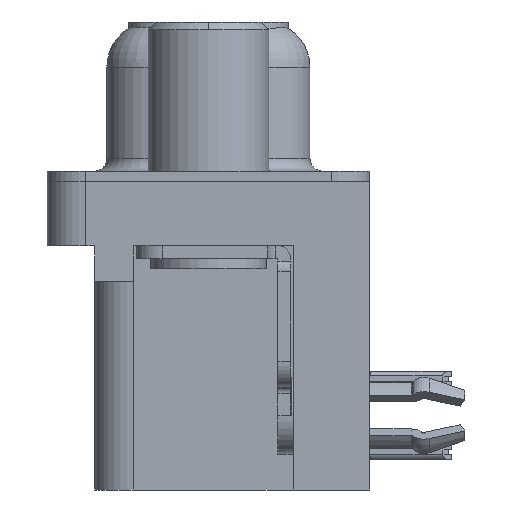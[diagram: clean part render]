
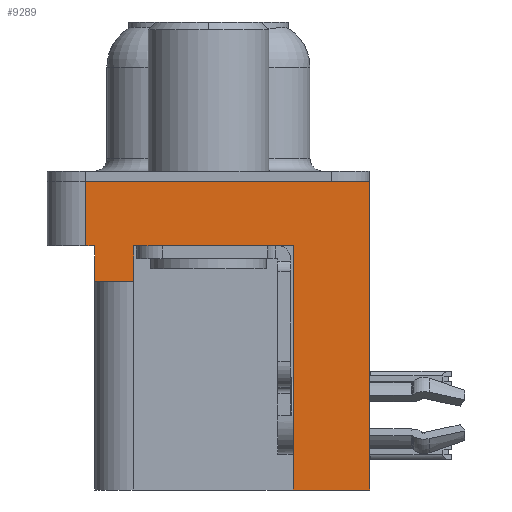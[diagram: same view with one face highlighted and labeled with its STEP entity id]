
A CAD part, left-side view. The second image highlights one B-rep face of the part: STEP entity #9289.
In plain terms, the highlighted planar face has unit normal (-1, 0, 0).
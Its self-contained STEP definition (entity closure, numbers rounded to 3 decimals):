
#329 = CARTESIAN_POINT ( 'NONE',  ( -2.935, -3.295, -12. ) ) ;
#2155 = CARTESIAN_POINT ( 'NONE',  ( -2.935, -6.275, -2.5 ) ) ;
#2458 = VECTOR ( 'NONE', #23388, 1000. ) ;
#2579 = LINE ( 'NONE', #3087, #22049 ) ;
#2972 = VERTEX_POINT ( 'NONE', #27534 ) ;
#3087 = CARTESIAN_POINT ( 'NONE',  ( -2.935, 4.425, -3.9 ) ) ;
#3257 = DIRECTION ( 'NONE',  ( 0., -1., 0. ) ) ;
#3308 = LINE ( 'NONE', #10274, #9508 ) ;
#3377 = VERTEX_POINT ( 'NONE', #11298 ) ;
#3486 = VECTOR ( 'NONE', #20382, 1000. ) ;
#4013 = VERTEX_POINT ( 'NONE', #5230 ) ;
#4302 = FACE_OUTER_BOUND ( 'NONE', #19098, .T. ) ;
#4414 = CARTESIAN_POINT ( 'NONE',  ( -2.935, -6.275, -2.5 ) ) ;
#4572 = DIRECTION ( 'NONE',  ( 0., -1., 0. ) ) ;
#4605 = EDGE_CURVE ( 'NONE', #3377, #26899, #18835, .T. ) ;
#5190 = VERTEX_POINT ( 'NONE', #20100 ) ;
#5230 = CARTESIAN_POINT ( 'NONE',  ( -2.935, 2.895, -2.5 ) ) ;
#5231 = VERTEX_POINT ( 'NONE', #13754 ) ;
#6147 = ORIENTED_EDGE ( 'NONE', *, *, #16762, .F. ) ;
#6730 = VERTEX_POINT ( 'NONE', #24211 ) ;
#7639 = VERTEX_POINT ( 'NONE', #17720 ) ;
#7646 = DIRECTION ( 'NONE',  ( 0., 0., 1. ) ) ;
#8039 = LINE ( 'NONE', #27539, #25761 ) ;
#8700 = EDGE_CURVE ( 'NONE', #5190, #7639, #2579, .T. ) ;
#8951 = CARTESIAN_POINT ( 'NONE',  ( -2.935, -6.275, 0. ) ) ;
#9289 = ADVANCED_FACE ( 'NONE', ( #4302 ), #15103, .T. ) ;
#9508 = VECTOR ( 'NONE', #16993, 1000. ) ;
#9856 = LINE ( 'NONE', #4414, #21050 ) ;
#10104 = CARTESIAN_POINT ( 'NONE',  ( -2.935, -3.295, -2.5 ) ) ;
#10274 = CARTESIAN_POINT ( 'NONE',  ( -2.935, 4.775, -2.5 ) ) ;
#10456 = DIRECTION ( 'NONE',  ( 0., 1., 0. ) ) ;
#10618 = ORIENTED_EDGE ( 'NONE', *, *, #15160, .T. ) ;
#10689 = DIRECTION ( 'NONE',  ( -1., 0., 0. ) ) ;
#11298 = CARTESIAN_POINT ( 'NONE',  ( -2.935, 4.775, 0. ) ) ;
#11533 = ORIENTED_EDGE ( 'NONE', *, *, #8700, .F. ) ;
#11577 = CARTESIAN_POINT ( 'NONE',  ( -2.935, -3.295, -12. ) ) ;
#12272 = DIRECTION ( 'NONE',  ( 0., 0., 1. ) ) ;
#12697 = EDGE_CURVE ( 'NONE', #5231, #27297, #23297, .T. ) ;
#12913 = VECTOR ( 'NONE', #4572, 1000. ) ;
#13441 = CARTESIAN_POINT ( 'NONE',  ( -2.935, 2.895, -3.9 ) ) ;
#13754 = CARTESIAN_POINT ( 'NONE',  ( -2.935, -6.275, -12. ) ) ;
#14406 = ORIENTED_EDGE ( 'NONE', *, *, #17805, .F. ) ;
#14420 = ORIENTED_EDGE ( 'NONE', *, *, #26349, .F. ) ;
#14487 = LINE ( 'NONE', #13441, #20780 ) ;
#14980 = LINE ( 'NONE', #2155, #2458 ) ;
#15103 = PLANE ( 'NONE',  #15478 ) ;
#15160 = EDGE_CURVE ( 'NONE', #2972, #4013, #14487, .T. ) ;
#15478 = AXIS2_PLACEMENT_3D ( 'NONE', #19555, #10689, #28091 ) ;
#15591 = EDGE_CURVE ( 'NONE', #5231, #26899, #14980, .T. ) ;
#15917 = ORIENTED_EDGE ( 'NONE', *, *, #21526, .T. ) ;
#15980 = VERTEX_POINT ( 'NONE', #10104 ) ;
#16762 = EDGE_CURVE ( 'NONE', #2972, #5190, #19349, .T. ) ;
#16815 = ORIENTED_EDGE ( 'NONE', *, *, #18184, .T. ) ;
#16993 = DIRECTION ( 'NONE',  ( 0., 0., 1. ) ) ;
#17197 = CARTESIAN_POINT ( 'NONE',  ( -2.935, 4.425, -3.9 ) ) ;
#17720 = CARTESIAN_POINT ( 'NONE',  ( -2.935, 4.425, -2.5 ) ) ;
#17805 = EDGE_CURVE ( 'NONE', #6730, #3377, #3308, .T. ) ;
#18184 = EDGE_CURVE ( 'NONE', #4013, #15980, #9856, .T. ) ;
#18629 = DIRECTION ( 'NONE',  ( 0., 0., 1. ) ) ;
#18835 = LINE ( 'NONE', #8951, #12913 ) ;
#19098 = EDGE_LOOP ( 'NONE', ( #26098, #14406, #15917, #11533, #6147, #10618, #16815, #14420, #26870, #21178 ) ) ;
#19349 = LINE ( 'NONE', #17197, #26626 ) ;
#19555 = CARTESIAN_POINT ( 'NONE',  ( -2.935, -6.275, -2.5 ) ) ;
#20100 = CARTESIAN_POINT ( 'NONE',  ( -2.935, 4.425, -3.9 ) ) ;
#20382 = DIRECTION ( 'NONE',  ( 0., 1., 0. ) ) ;
#20780 = VECTOR ( 'NONE', #12272, 1000. ) ;
#20916 = LINE ( 'NONE', #23172, #25705 ) ;
#21050 = VECTOR ( 'NONE', #22208, 1000. ) ;
#21178 = ORIENTED_EDGE ( 'NONE', *, *, #15591, .T. ) ;
#21526 = EDGE_CURVE ( 'NONE', #6730, #7639, #20916, .T. ) ;
#22049 = VECTOR ( 'NONE', #18629, 1000. ) ;
#22208 = DIRECTION ( 'NONE',  ( 0., -1., 0. ) ) ;
#23172 = CARTESIAN_POINT ( 'NONE',  ( -2.935, -6.275, -2.5 ) ) ;
#23297 = LINE ( 'NONE', #11577, #3486 ) ;
#23388 = DIRECTION ( 'NONE',  ( 0., 0., 1. ) ) ;
#24211 = CARTESIAN_POINT ( 'NONE',  ( -2.935, 4.775, -2.5 ) ) ;
#25259 = CARTESIAN_POINT ( 'NONE',  ( -2.935, -6.275, 0. ) ) ;
#25705 = VECTOR ( 'NONE', #3257, 1000. ) ;
#25761 = VECTOR ( 'NONE', #7646, 1000. ) ;
#26098 = ORIENTED_EDGE ( 'NONE', *, *, #4605, .F. ) ;
#26349 = EDGE_CURVE ( 'NONE', #27297, #15980, #8039, .T. ) ;
#26626 = VECTOR ( 'NONE', #10456, 1000. ) ;
#26870 = ORIENTED_EDGE ( 'NONE', *, *, #12697, .F. ) ;
#26899 = VERTEX_POINT ( 'NONE', #25259 ) ;
#27297 = VERTEX_POINT ( 'NONE', #329 ) ;
#27534 = CARTESIAN_POINT ( 'NONE',  ( -2.935, 2.895, -3.9 ) ) ;
#27539 = CARTESIAN_POINT ( 'NONE',  ( -2.935, -3.295, -12. ) ) ;
#28091 = DIRECTION ( 'NONE',  ( 0., 0., 1. ) ) ;
